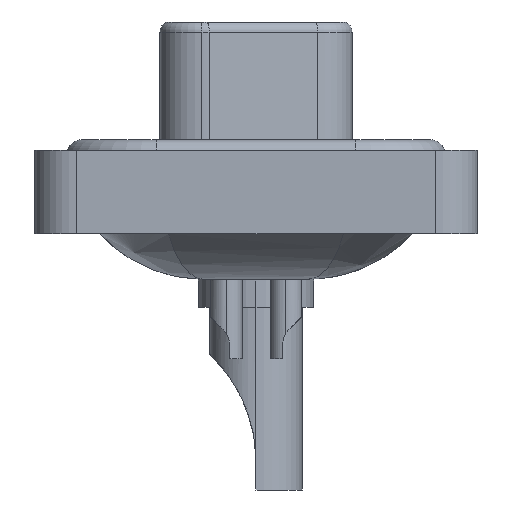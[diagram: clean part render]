
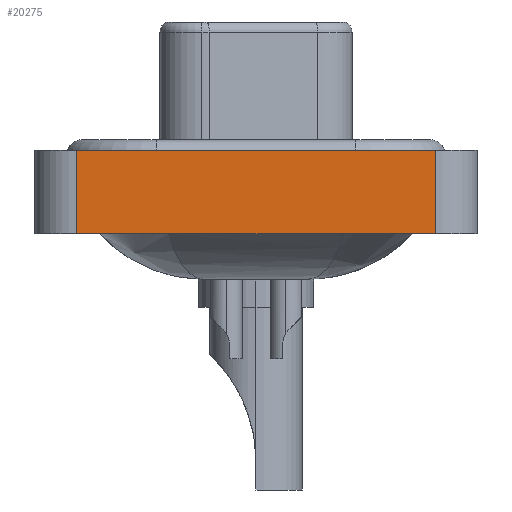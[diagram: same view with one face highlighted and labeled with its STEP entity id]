
A CAD part, left-side view. The second image highlights one B-rep face of the part: STEP entity #20275.
In plain terms, the highlighted planar face has unit normal (-1, 0, 0).
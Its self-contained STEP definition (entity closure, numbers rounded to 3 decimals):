
#864 = ORIENTED_EDGE ( 'NONE', *, *, #3626, .T. ) ;
#1080 = VERTEX_POINT ( 'NONE', #2386 ) ;
#1259 = AXIS2_PLACEMENT_3D ( 'NONE', #5472, #12043, #2295 ) ;
#1400 = ORIENTED_EDGE ( 'NONE', *, *, #13814, .F. ) ;
#1558 = VERTEX_POINT ( 'NONE', #11805 ) ;
#2161 = LINE ( 'NONE', #14912, #14392 ) ;
#2295 = DIRECTION ( 'NONE',  ( 0., 0., 1. ) ) ;
#2386 = CARTESIAN_POINT ( 'NONE',  ( -7.3, -8.55, 0.4 ) ) ;
#2676 = DIRECTION ( 'NONE',  ( 0., -1., 0. ) ) ;
#3076 = CARTESIAN_POINT ( 'NONE',  ( -7.3, -8.55, -3.6 ) ) ;
#3455 = LINE ( 'NONE', #14506, #3644 ) ;
#3626 = EDGE_CURVE ( 'NONE', #13660, #9206, #17435, .T. ) ;
#3644 = VECTOR ( 'NONE', #19493, 1000. ) ;
#3808 = CARTESIAN_POINT ( 'NONE',  ( -7.3, 8.55, -3.6 ) ) ;
#4756 = CARTESIAN_POINT ( 'NONE',  ( -7.3, -8.55, -3.6 ) ) ;
#4855 = CARTESIAN_POINT ( 'NONE',  ( -7.3, 8.55, -3.6 ) ) ;
#5472 = CARTESIAN_POINT ( 'NONE',  ( -7.3, -8.55, -3.6 ) ) ;
#5729 = ORIENTED_EDGE ( 'NONE', *, *, #17800, .F. ) ;
#6768 = VECTOR ( 'NONE', #2676, 1000. ) ;
#7225 = LINE ( 'NONE', #3808, #20267 ) ;
#9206 = VERTEX_POINT ( 'NONE', #4756 ) ;
#11727 = FACE_OUTER_BOUND ( 'NONE', #13683, .T. ) ;
#11805 = CARTESIAN_POINT ( 'NONE',  ( -7.3, 8.55, 0.4 ) ) ;
#12043 = DIRECTION ( 'NONE',  ( -1., 0., 0. ) ) ;
#13660 = VERTEX_POINT ( 'NONE', #4855 ) ;
#13683 = EDGE_LOOP ( 'NONE', ( #19810, #5729, #1400, #864 ) ) ;
#13734 = DIRECTION ( 'NONE',  ( 0., -1., 0. ) ) ;
#13814 = EDGE_CURVE ( 'NONE', #13660, #1558, #7225, .T. ) ;
#14392 = VECTOR ( 'NONE', #13734, 1000. ) ;
#14506 = CARTESIAN_POINT ( 'NONE',  ( -7.3, -8.55, -3.6 ) ) ;
#14912 = CARTESIAN_POINT ( 'NONE',  ( -7.3, -8.55, 0.4 ) ) ;
#16985 = DIRECTION ( 'NONE',  ( 0., 0., 1. ) ) ;
#17435 = LINE ( 'NONE', #3076, #6768 ) ;
#17800 = EDGE_CURVE ( 'NONE', #1558, #1080, #2161, .T. ) ;
#19493 = DIRECTION ( 'NONE',  ( 0., 0., 1. ) ) ;
#19810 = ORIENTED_EDGE ( 'NONE', *, *, #20127, .T. ) ;
#20037 = PLANE ( 'NONE',  #1259 ) ;
#20127 = EDGE_CURVE ( 'NONE', #9206, #1080, #3455, .T. ) ;
#20267 = VECTOR ( 'NONE', #16985, 1000. ) ;
#20275 = ADVANCED_FACE ( 'NONE', ( #11727 ), #20037, .T. ) ;
